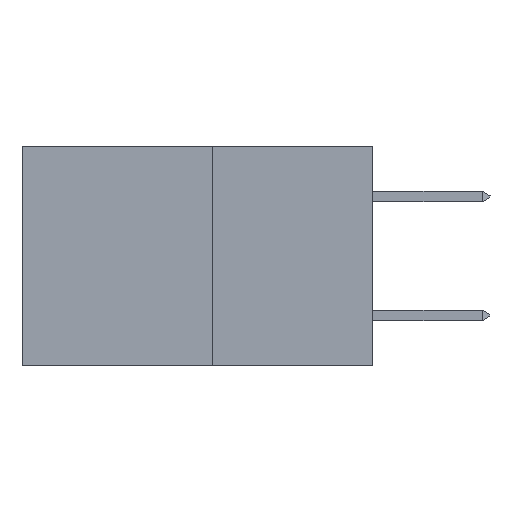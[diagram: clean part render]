
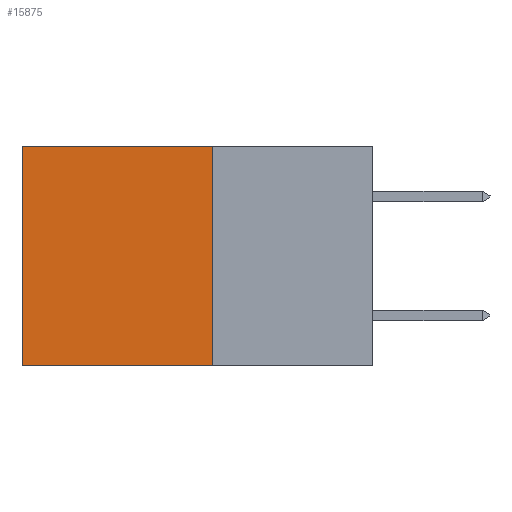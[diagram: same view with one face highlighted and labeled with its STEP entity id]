
A CAD part, left-side view. The second image highlights one B-rep face of the part: STEP entity #15875.
In plain terms, the highlighted planar face has unit normal (-1, 0, 0).
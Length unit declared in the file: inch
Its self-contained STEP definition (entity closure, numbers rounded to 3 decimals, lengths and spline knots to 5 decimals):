
#196 = LINE ( 'NONE', #6924, #12238 ) ;
#691 = CARTESIAN_POINT ( 'NONE',  ( 0.277, 0.27, -0.37 ) ) ;
#1121 = VECTOR ( 'NONE', #23111, 39.37008 ) ;
#1870 = DIRECTION ( 'NONE',  ( 0., 1., 0. ) ) ;
#2352 = PLANE ( 'NONE',  #14723 ) ;
#2412 = ORIENTED_EDGE ( 'NONE', *, *, #28488, .F. ) ;
#2601 = CARTESIAN_POINT ( 'NONE',  ( 0.277, 0.27, 0. ) ) ;
#5196 = ORIENTED_EDGE ( 'NONE', *, *, #19458, .T. ) ;
#5425 = ORIENTED_EDGE ( 'NONE', *, *, #8869, .T. ) ;
#6851 = DIRECTION ( 'NONE',  ( 0., 0., -1. ) ) ;
#6924 = CARTESIAN_POINT ( 'NONE',  ( 0.277, 0.59, -0.37 ) ) ;
#6968 = LINE ( 'NONE', #28965, #12536 ) ;
#8346 = LINE ( 'NONE', #8696, #1121 ) ;
#8696 = CARTESIAN_POINT ( 'NONE',  ( 0.277, 0.27, -0.37 ) ) ;
#8869 = EDGE_CURVE ( 'NONE', #18255, #29278, #196, .T. ) ;
#9768 = CARTESIAN_POINT ( 'NONE',  ( 0.277, 0.59, -0.37 ) ) ;
#11443 = CARTESIAN_POINT ( 'NONE',  ( 0.277, 0.27, 0. ) ) ;
#12019 = DIRECTION ( 'NONE',  ( 1., 0., 0. ) ) ;
#12238 = VECTOR ( 'NONE', #6851, 39.37008 ) ;
#12536 = VECTOR ( 'NONE', #16788, 39.37008 ) ;
#14723 = AXIS2_PLACEMENT_3D ( 'NONE', #24070, #12019, #28985 ) ;
#15241 = VERTEX_POINT ( 'NONE', #691 ) ;
#15875 = ADVANCED_FACE ( 'NONE', ( #25527 ), #2352, .F. ) ;
#16788 = DIRECTION ( 'NONE',  ( 0., 0., -1. ) ) ;
#18255 = VERTEX_POINT ( 'NONE', #30432 ) ;
#19045 = ORIENTED_EDGE ( 'NONE', *, *, #30220, .F. ) ;
#19458 = EDGE_CURVE ( 'NONE', #27537, #18255, #30977, .T. ) ;
#23111 = DIRECTION ( 'NONE',  ( 0., 1., 0. ) ) ;
#24070 = CARTESIAN_POINT ( 'NONE',  ( 0.277, 0.27, -0.37 ) ) ;
#24493 = VECTOR ( 'NONE', #1870, 39.37008 ) ;
#24738 = EDGE_LOOP ( 'NONE', ( #5425, #19045, #2412, #5196 ) ) ;
#25527 = FACE_OUTER_BOUND ( 'NONE', #24738, .T. ) ;
#27537 = VERTEX_POINT ( 'NONE', #2601 ) ;
#28488 = EDGE_CURVE ( 'NONE', #27537, #15241, #6968, .T. ) ;
#28965 = CARTESIAN_POINT ( 'NONE',  ( 0.277, 0.27, -0.37 ) ) ;
#28985 = DIRECTION ( 'NONE',  ( 0., 0., -1. ) ) ;
#29278 = VERTEX_POINT ( 'NONE', #9768 ) ;
#30220 = EDGE_CURVE ( 'NONE', #15241, #29278, #8346, .T. ) ;
#30432 = CARTESIAN_POINT ( 'NONE',  ( 0.277, 0.59, 0. ) ) ;
#30977 = LINE ( 'NONE', #11443, #24493 ) ;
